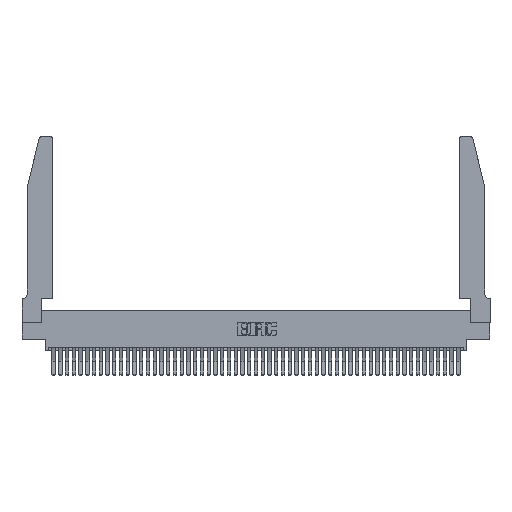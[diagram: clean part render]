
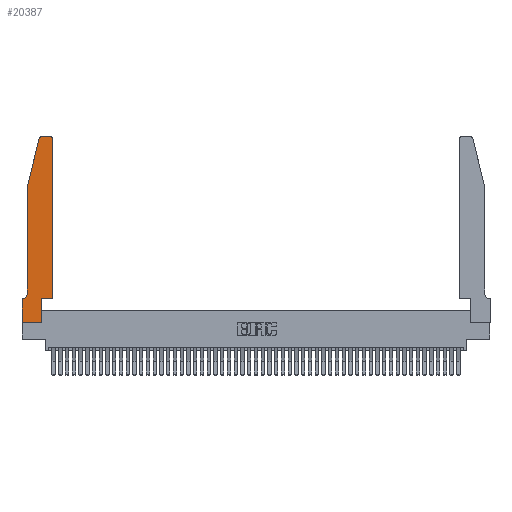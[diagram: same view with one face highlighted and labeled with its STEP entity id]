
A CAD part, top view. The second image highlights one B-rep face of the part: STEP entity #20387.
In plain terms, the highlighted planar face has unit normal (0, 0, 1).
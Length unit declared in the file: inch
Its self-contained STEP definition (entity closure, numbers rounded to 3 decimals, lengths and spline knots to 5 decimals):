
#252 = CARTESIAN_POINT ( 'NONE',  ( 0.2865, 0.35, 0.37 ) ) ;
#361 = ORIENTED_EDGE ( 'NONE', *, *, #2399, .T. ) ;
#2115 = VERTEX_POINT ( 'NONE', #31931 ) ;
#2134 = EDGE_CURVE ( 'NONE', #41253, #49192, #19116, .T. ) ;
#2399 = EDGE_CURVE ( 'NONE', #34156, #8756, #35497, .T. ) ;
#2542 = CARTESIAN_POINT ( 'NONE',  ( 0.0755, 0.42, 0.37 ) ) ;
#3349 = LINE ( 'NONE', #20980, #12462 ) ;
#3695 = CIRCLE ( 'NONE', #44646, 0.03 ) ;
#4510 = EDGE_CURVE ( 'NONE', #20231, #21788, #14012, .T. ) ;
#4615 = DIRECTION ( 'NONE',  ( 1., 0., 0. ) ) ;
#5092 = EDGE_CURVE ( 'NONE', #31896, #15982, #12170, .T. ) ;
#5643 = DIRECTION ( 'NONE',  ( -1., 0., 0. ) ) ;
#6564 = EDGE_CURVE ( 'NONE', #21788, #41253, #42653, .T. ) ;
#7388 = LINE ( 'NONE', #8226, #16494 ) ;
#7625 = EDGE_CURVE ( 'NONE', #42503, #2115, #3695, .T. ) ;
#8226 = CARTESIAN_POINT ( 'NONE',  ( 0.0755, 2., 0.37 ) ) ;
#8756 = VERTEX_POINT ( 'NONE', #13703 ) ;
#9909 = DIRECTION ( 'NONE',  ( 1., 0., 0. ) ) ;
#10512 = ORIENTED_EDGE ( 'NONE', *, *, #2134, .T. ) ;
#11651 = AXIS2_PLACEMENT_3D ( 'NONE', #21132, #13442, #5643 ) ;
#11831 = VERTEX_POINT ( 'NONE', #23722 ) ;
#12170 = CIRCLE ( 'NONE', #11651, 0.07 ) ;
#12462 = VECTOR ( 'NONE', #47620, 39.37008 ) ;
#13442 = DIRECTION ( 'NONE',  ( 0., 0., -1. ) ) ;
#13703 = CARTESIAN_POINT ( 'NONE',  ( 0.4205, 2.75, 0.37 ) ) ;
#14012 = LINE ( 'NONE', #19567, #31091 ) ;
#14647 = DIRECTION ( 'NONE',  ( 1., 0., 0. ) ) ;
#14678 = ORIENTED_EDGE ( 'NONE', *, *, #4510, .T. ) ;
#15035 = DIRECTION ( 'NONE',  ( -1., 0., 0. ) ) ;
#15866 = DIRECTION ( 'NONE',  ( 0., 0., 1. ) ) ;
#15872 = EDGE_LOOP ( 'NONE', ( #35675, #31854, #48777, #25119, #32863, #42689, #36940, #14678, #18202, #10512, #29131, #361 ) ) ;
#15982 = VERTEX_POINT ( 'NONE', #48309 ) ;
#16353 = DIRECTION ( 'NONE',  ( 0., -1., 0. ) ) ;
#16494 = VECTOR ( 'NONE', #16353, 39.37008 ) ;
#16707 = LINE ( 'NONE', #22970, #49472 ) ;
#16866 = DIRECTION ( 'NONE',  ( -0.239, -0.971, 0. ) ) ;
#17793 = AXIS2_PLACEMENT_3D ( 'NONE', #22364, #37978, #14647 ) ;
#18202 = ORIENTED_EDGE ( 'NONE', *, *, #6564, .T. ) ;
#18707 = DIRECTION ( 'NONE',  ( 0., -1., 0. ) ) ;
#19116 = LINE ( 'NONE', #43443, #42183 ) ;
#19567 = CARTESIAN_POINT ( 'NONE',  ( 0., 0., 0.37 ) ) ;
#19834 = EDGE_CURVE ( 'NONE', #2115, #26274, #33089, .T. ) ;
#20010 = CARTESIAN_POINT ( 'NONE',  ( 0.0755, 0.35, 0.37 ) ) ;
#20191 = CARTESIAN_POINT ( 'NONE',  ( 0.4505, 0.35, 0.37 ) ) ;
#20231 = VERTEX_POINT ( 'NONE', #33983 ) ;
#20387 = ADVANCED_FACE ( 'NONE', ( #26344 ), #21184, .T. ) ;
#20965 = DIRECTION ( 'NONE',  ( 0., 1., 0. ) ) ;
#20980 = CARTESIAN_POINT ( 'NONE',  ( 0.2605, 2.75, 0.37 ) ) ;
#21132 = CARTESIAN_POINT ( 'NONE',  ( 0.0055, 0.42, 0.37 ) ) ;
#21162 = EDGE_CURVE ( 'NONE', #26274, #31896, #7388, .T. ) ;
#21184 = PLANE ( 'NONE',  #24501 ) ;
#21788 = VERTEX_POINT ( 'NONE', #30808 ) ;
#21808 = VECTOR ( 'NONE', #15035, 39.37008 ) ;
#22364 = CARTESIAN_POINT ( 'NONE',  ( 0.4205, 2.72, 0.37 ) ) ;
#22970 = CARTESIAN_POINT ( 'NONE',  ( 0., 0., 0.37 ) ) ;
#23375 = CARTESIAN_POINT ( 'NONE',  ( 0.284, 2.72, 0.37 ) ) ;
#23476 = EDGE_CURVE ( 'NONE', #15982, #11831, #46651, .T. ) ;
#23722 = CARTESIAN_POINT ( 'NONE',  ( 0., 0.35, 0.37 ) ) ;
#24501 = AXIS2_PLACEMENT_3D ( 'NONE', #47649, #44435, #24915 ) ;
#24915 = DIRECTION ( 'NONE',  ( 1., 0., 0. ) ) ;
#25119 = ORIENTED_EDGE ( 'NONE', *, *, #21162, .T. ) ;
#25869 = DIRECTION ( 'NONE',  ( 0., 1., 0. ) ) ;
#26274 = VERTEX_POINT ( 'NONE', #41127 ) ;
#26344 = FACE_OUTER_BOUND ( 'NONE', #15872, .T. ) ;
#29131 = ORIENTED_EDGE ( 'NONE', *, *, #44069, .T. ) ;
#30048 = EDGE_CURVE ( 'NONE', #11831, #20231, #16707, .T. ) ;
#30194 = VECTOR ( 'NONE', #20965, 39.37008 ) ;
#30808 = CARTESIAN_POINT ( 'NONE',  ( 0.2865, 0., 0.37 ) ) ;
#31091 = VECTOR ( 'NONE', #4615, 39.37008 ) ;
#31854 = ORIENTED_EDGE ( 'NONE', *, *, #7625, .T. ) ;
#31896 = VERTEX_POINT ( 'NONE', #2542 ) ;
#31931 = CARTESIAN_POINT ( 'NONE',  ( 0.25487, 2.72718, 0.37 ) ) ;
#32713 = CARTESIAN_POINT ( 'NONE',  ( 0.4505, 2.72, 0.37 ) ) ;
#32863 = ORIENTED_EDGE ( 'NONE', *, *, #5092, .T. ) ;
#33089 = LINE ( 'NONE', #48091, #38549 ) ;
#33563 = VECTOR ( 'NONE', #25869, 39.37008 ) ;
#33983 = CARTESIAN_POINT ( 'NONE',  ( 0., 0., 0.37 ) ) ;
#34156 = VERTEX_POINT ( 'NONE', #32713 ) ;
#35497 = CIRCLE ( 'NONE', #17793, 0.03 ) ;
#35675 = ORIENTED_EDGE ( 'NONE', *, *, #38575, .T. ) ;
#36940 = ORIENTED_EDGE ( 'NONE', *, *, #30048, .T. ) ;
#37741 = CARTESIAN_POINT ( 'NONE',  ( 0.284, 2.75, 0.37 ) ) ;
#37978 = DIRECTION ( 'NONE',  ( 0., 0., 1. ) ) ;
#38549 = VECTOR ( 'NONE', #16866, 39.37008 ) ;
#38575 = EDGE_CURVE ( 'NONE', #8756, #42503, #3349, .T. ) ;
#41127 = CARTESIAN_POINT ( 'NONE',  ( 0.0755, 2., 0.37 ) ) ;
#41253 = VERTEX_POINT ( 'NONE', #252 ) ;
#41648 = CARTESIAN_POINT ( 'NONE',  ( 0.2865, 0.35, 0.37 ) ) ;
#41698 = LINE ( 'NONE', #48092, #30194 ) ;
#42183 = VECTOR ( 'NONE', #9909, 39.37008 ) ;
#42503 = VERTEX_POINT ( 'NONE', #37741 ) ;
#42653 = LINE ( 'NONE', #41648, #33563 ) ;
#42689 = ORIENTED_EDGE ( 'NONE', *, *, #23476, .T. ) ;
#43043 = DIRECTION ( 'NONE',  ( 1., 0., 0. ) ) ;
#43443 = CARTESIAN_POINT ( 'NONE',  ( 0.4505, 0.35, 0.37 ) ) ;
#44069 = EDGE_CURVE ( 'NONE', #49192, #34156, #41698, .T. ) ;
#44435 = DIRECTION ( 'NONE',  ( 0., 0., 1. ) ) ;
#44646 = AXIS2_PLACEMENT_3D ( 'NONE', #23375, #15866, #43043 ) ;
#46651 = LINE ( 'NONE', #20010, #21808 ) ;
#47620 = DIRECTION ( 'NONE',  ( -1., 0., 0. ) ) ;
#47649 = CARTESIAN_POINT ( 'NONE',  ( 0., 0.35, 0.37 ) ) ;
#48091 = CARTESIAN_POINT ( 'NONE',  ( 0.0755, 2., 0.37 ) ) ;
#48092 = CARTESIAN_POINT ( 'NONE',  ( 0.4505, 0.35, 0.37 ) ) ;
#48309 = CARTESIAN_POINT ( 'NONE',  ( 0.0055, 0.35, 0.37 ) ) ;
#48777 = ORIENTED_EDGE ( 'NONE', *, *, #19834, .T. ) ;
#49192 = VERTEX_POINT ( 'NONE', #20191 ) ;
#49472 = VECTOR ( 'NONE', #18707, 39.37008 ) ;
